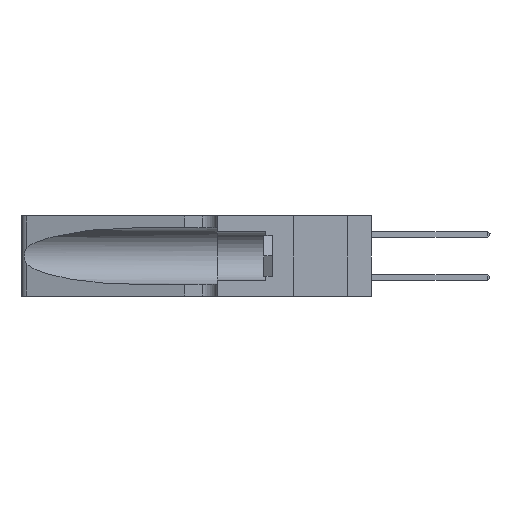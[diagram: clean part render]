
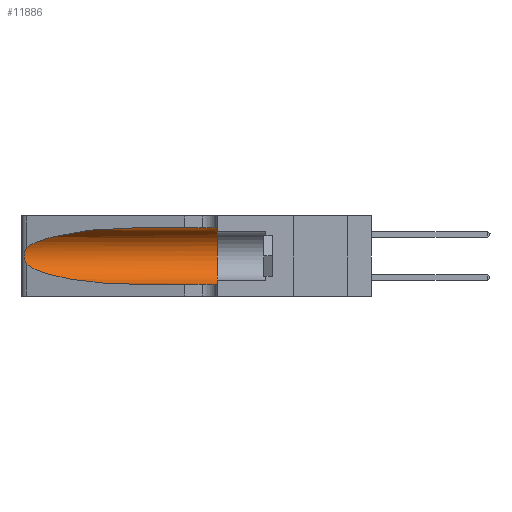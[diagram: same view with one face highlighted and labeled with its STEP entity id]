
A CAD part, left-side view. The second image highlights one B-rep face of the part: STEP entity #11886.
In plain terms, the highlighted cylindrical face has radius 3.308 mm (diameter 6.617 mm), a partial arc.
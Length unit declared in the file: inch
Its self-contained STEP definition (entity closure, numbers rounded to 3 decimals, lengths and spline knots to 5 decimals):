
#177 = CARTESIAN_POINT ( 'NONE',  ( 0.25555, 1.22993, 0.14849 ) ) ;
#837 = ORIENTED_EDGE ( 'NONE', *, *, #13604, .T. ) ;
#1065 =( BOUNDED_CURVE ( )  B_SPLINE_CURVE ( 3, ( #31054, #31181, #10619, #19911 ),
 .UNSPECIFIED., .F., .T. ) 
 B_SPLINE_CURVE_WITH_KNOTS ( ( 4, 4 ),
 ( 1.5708, 2.84003 ),
 .UNSPECIFIED. ) 
 CURVE ( )  GEOMETRIC_REPRESENTATION_ITEM ( )  RATIONAL_B_SPLINE_CURVE ( ( 1., 0.87, 0.87, 1. ) ) 
 REPRESENTATION_ITEM ( '' )  );
#3296 = AXIS2_PLACEMENT_3D ( 'NONE', #19880, #17975, #37294 ) ;
#3851 = VERTEX_POINT ( 'NONE', #37803 ) ;
#5058 = CARTESIAN_POINT ( 'NONE',  ( 0.18966, 0.96281, 0.05475 ) ) ;
#5717 = CARTESIAN_POINT ( 'NONE',  ( 0.25639, 1.23186, 0.15144 ) ) ;
#6119 = CARTESIAN_POINT ( 'NONE',  ( 0.25487, 1.22718, 0.22369 ) ) ;
#7013 =( BOUNDED_CURVE ( )  B_SPLINE_CURVE ( 3, ( #29940, #14238, #5058, #32919 ),
 .UNSPECIFIED., .F., .T. ) 
 B_SPLINE_CURVE_WITH_KNOTS ( ( 4, 4 ),
 ( 3.44316, 4.71239 ),
 .UNSPECIFIED. ) 
 CURVE ( )  GEOMETRIC_REPRESENTATION_ITEM ( )  RATIONAL_B_SPLINE_CURVE ( ( 1., 0.87, 0.87, 1. ) ) 
 REPRESENTATION_ITEM ( '' )  );
#7533 = CARTESIAN_POINT ( 'NONE',  ( 0.1305, 1.61858, 0.05475 ) ) ;
#8988 = CARTESIAN_POINT ( 'NONE',  ( 0.25854, 1.2359, 0.20912 ) ) ;
#10619 = CARTESIAN_POINT ( 'NONE',  ( 0.2373, 1.15595, 0.28018 ) ) ;
#10728 = ORIENTED_EDGE ( 'NONE', *, *, #25204, .F. ) ;
#11580 = CARTESIAN_POINT ( 'NONE',  ( 0.1305, 0.35, 0.185 ) ) ;
#11886 = ADVANCED_FACE ( 'NONE', ( #24432 ), #22464, .F. ) ;
#12193 = CARTESIAN_POINT ( 'NONE',  ( 0.26018, 1.23835, 0.19895 ) ) ;
#12341 = VECTOR ( 'NONE', #32103, 39.37008 ) ;
#12453 = CARTESIAN_POINT ( 'NONE',  ( 0.25856, 1.23593, 0.16098 ) ) ;
#12986 = CARTESIAN_POINT ( 'NONE',  ( 0.1305, 0.72297, 0.05475 ) ) ;
#13604 = EDGE_CURVE ( 'NONE', #21759, #31716, #1065, .T. ) ;
#14238 = CARTESIAN_POINT ( 'NONE',  ( 0.2373, 1.15595, 0.08982 ) ) ;
#15140 = CARTESIAN_POINT ( 'NONE',  ( 0.26075, 1.23896, 0.19203 ) ) ;
#15222 = LINE ( 'NONE', #32565, #25770 ) ;
#15278 = CARTESIAN_POINT ( 'NONE',  ( 0.26075, 1.23896, 0.178 ) ) ;
#16361 = ORIENTED_EDGE ( 'NONE', *, *, #36663, .T. ) ;
#17314 = CARTESIAN_POINT ( 'NONE',  ( 0.25487, 1.22718, 0.14631 ) ) ;
#17749 = DIRECTION ( 'NONE',  ( 0., 1., 0. ) ) ;
#17975 = DIRECTION ( 'NONE',  ( 0., -1., 0. ) ) ;
#18093 = LINE ( 'NONE', #7533, #12341 ) ;
#18259 = CARTESIAN_POINT ( 'NONE',  ( 0.25555, 1.22994, 0.2215 ) ) ;
#18671 = CIRCLE ( 'NONE', #37962, 0.13025 ) ;
#19815 = VERTEX_POINT ( 'NONE', #12986 ) ;
#19880 = CARTESIAN_POINT ( 'NONE',  ( 0.1305, 1.61858, 0.185 ) ) ;
#19911 = CARTESIAN_POINT ( 'NONE',  ( 0.25487, 1.22718, 0.22369 ) ) ;
#21199 = CARTESIAN_POINT ( 'NONE',  ( 0.25487, 1.22718, 0.14631 ) ) ;
#21743 = ORIENTED_EDGE ( 'NONE', *, *, #23166, .T. ) ;
#21759 = VERTEX_POINT ( 'NONE', #24462 ) ;
#22464 = CYLINDRICAL_SURFACE ( 'NONE', #3296, 0.13025 ) ;
#22557 = CARTESIAN_POINT ( 'NONE',  ( 0.25487, 1.22718, 0.22369 ) ) ;
#22890 = VERTEX_POINT ( 'NONE', #17314 ) ;
#23166 = EDGE_CURVE ( 'NONE', #19815, #3851, #18093, .T. ) ;
#24432 = FACE_OUTER_BOUND ( 'NONE', #32895, .T. ) ;
#24462 = CARTESIAN_POINT ( 'NONE',  ( 0.1305, 0.72297, 0.31525 ) ) ;
#25204 = EDGE_CURVE ( 'NONE', #34265, #3851, #18671, .T. ) ;
#25770 = VECTOR ( 'NONE', #25994, 39.37008 ) ;
#25994 = DIRECTION ( 'NONE',  ( 0., -1., 0. ) ) ;
#27365 = CARTESIAN_POINT ( 'NONE',  ( 0.26017, 1.23833, 0.17102 ) ) ;
#27652 = ORIENTED_EDGE ( 'NONE', *, *, #39023, .F. ) ;
#28849 = EDGE_CURVE ( 'NONE', #22890, #19815, #7013, .T. ) ;
#29940 = CARTESIAN_POINT ( 'NONE',  ( 0.25487, 1.22718, 0.14631 ) ) ;
#30565 = CARTESIAN_POINT ( 'NONE',  ( 0.25639, 1.23184, 0.21858 ) ) ;
#30618 = B_SPLINE_CURVE_WITH_KNOTS ( 'NONE', 3,
 ( #6119, #18259, #30565, #33550, #8988, #12193, #15140, #15278, #27365, #12453, #36741, #5717, #177, #21199 ),
 .UNSPECIFIED., .F., .F.,
 ( 4, 2, 2, 2, 2, 2, 4 ),
 ( 0., 0.00027, 0.00053, 0.00107, 0.0016, 0.00187, 0.00214 ),
 .UNSPECIFIED. ) ;
#30895 = ORIENTED_EDGE ( 'NONE', *, *, #28849, .T. ) ;
#31054 = CARTESIAN_POINT ( 'NONE',  ( 0.1305, 0.72297, 0.31525 ) ) ;
#31181 = CARTESIAN_POINT ( 'NONE',  ( 0.18966, 0.96281, 0.31525 ) ) ;
#31716 = VERTEX_POINT ( 'NONE', #22557 ) ;
#32103 = DIRECTION ( 'NONE',  ( 0., -1., 0. ) ) ;
#32167 = CARTESIAN_POINT ( 'NONE',  ( 0.1305, 0.35, 0.31525 ) ) ;
#32565 = CARTESIAN_POINT ( 'NONE',  ( 0.1305, 1.61858, 0.31525 ) ) ;
#32895 = EDGE_LOOP ( 'NONE', ( #837, #16361, #30895, #21743, #10728, #27652 ) ) ;
#32919 = CARTESIAN_POINT ( 'NONE',  ( 0.1305, 0.72297, 0.05475 ) ) ;
#33045 = DIRECTION ( 'NONE',  ( 0., 0., 1. ) ) ;
#33550 = CARTESIAN_POINT ( 'NONE',  ( 0.25787, 1.23484, 0.2124 ) ) ;
#34265 = VERTEX_POINT ( 'NONE', #32167 ) ;
#36663 = EDGE_CURVE ( 'NONE', #31716, #22890, #30618, .T. ) ;
#36741 = CARTESIAN_POINT ( 'NONE',  ( 0.25789, 1.23486, 0.15765 ) ) ;
#37294 = DIRECTION ( 'NONE',  ( 0., 0., -1. ) ) ;
#37803 = CARTESIAN_POINT ( 'NONE',  ( 0.1305, 0.35, 0.05475 ) ) ;
#37962 = AXIS2_PLACEMENT_3D ( 'NONE', #11580, #17749, #33045 ) ;
#39023 = EDGE_CURVE ( 'NONE', #21759, #34265, #15222, .T. ) ;
